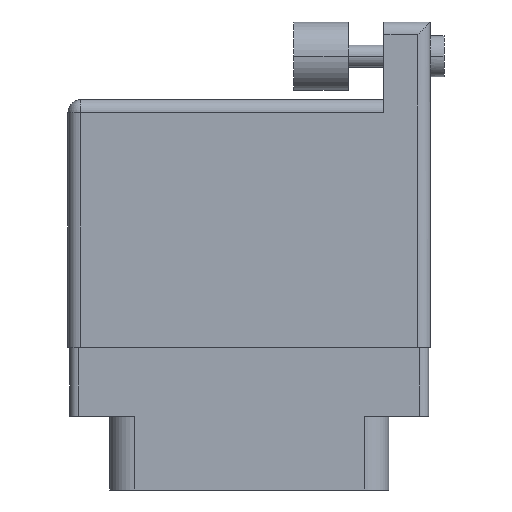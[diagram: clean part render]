
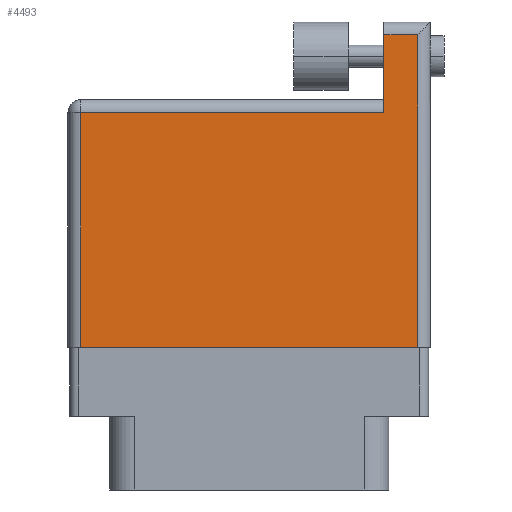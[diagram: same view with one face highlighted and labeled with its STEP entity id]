
A CAD part, front view. The second image highlights one B-rep face of the part: STEP entity #4493.
In plain terms, the highlighted face is planar.
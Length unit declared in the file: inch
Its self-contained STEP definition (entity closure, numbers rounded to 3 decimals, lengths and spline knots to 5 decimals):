
#418 = VECTOR ( 'NONE', #1665, 39.37008 ) ;
#433 = VERTEX_POINT ( 'NONE', #20289 ) ;
#471 = VECTOR ( 'NONE', #10760, 39.37008 ) ;
#1665 = DIRECTION ( 'NONE',  ( 0., 1., 0. ) ) ;
#1786 = CARTESIAN_POINT ( 'NONE',  ( 0.047, 0.859, 0. ) ) ;
#2271 = EDGE_CURVE ( 'NONE', #8817, #2777, #4031, .T. ) ;
#2643 = DIRECTION ( 'NONE',  ( 0., 0., -1. ) ) ;
#2777 = VERTEX_POINT ( 'NONE', #15949 ) ;
#2912 = VECTOR ( 'NONE', #10332, 39.37008 ) ;
#3326 = CARTESIAN_POINT ( 'NONE',  ( 1.278, 1.143, 0. ) ) ;
#3632 = ORIENTED_EDGE ( 'NONE', *, *, #8493, .T. ) ;
#4031 = LINE ( 'NONE', #20857, #2912 ) ;
#4182 = ORIENTED_EDGE ( 'NONE', *, *, #2271, .T. ) ;
#4493 = ADVANCED_FACE ( 'NONE', ( #7627 ), #17918, .F. ) ;
#5106 = LINE ( 'NONE', #11848, #418 ) ;
#5687 = ORIENTED_EDGE ( 'NONE', *, *, #17896, .T. ) ;
#5809 = LINE ( 'NONE', #12546, #18740 ) ;
#6690 = CARTESIAN_POINT ( 'NONE',  ( 1.155, 1.19, 0. ) ) ;
#7219 = CARTESIAN_POINT ( 'NONE',  ( 0.047, 0., 0. ) ) ;
#7345 = LINE ( 'NONE', #20630, #471 ) ;
#7584 = EDGE_LOOP ( 'NONE', ( #4182, #20610, #12353, #5687, #3632, #17560 ) ) ;
#7627 = FACE_OUTER_BOUND ( 'NONE', #7584, .T. ) ;
#8493 = EDGE_CURVE ( 'NONE', #10558, #19634, #5809, .T. ) ;
#8817 = VERTEX_POINT ( 'NONE', #7219 ) ;
#9152 = AXIS2_PLACEMENT_3D ( 'NONE', #15817, #2643, #10718 ) ;
#9871 = VERTEX_POINT ( 'NONE', #3326 ) ;
#10332 = DIRECTION ( 'NONE',  ( 1., 0., 0. ) ) ;
#10333 = VECTOR ( 'NONE', #11768, 39.37008 ) ;
#10558 = VERTEX_POINT ( 'NONE', #16752 ) ;
#10718 = DIRECTION ( 'NONE',  ( -1., 0., 0. ) ) ;
#10760 = DIRECTION ( 'NONE',  ( -1., 0., 0. ) ) ;
#11133 = EDGE_CURVE ( 'NONE', #2777, #9871, #5106, .T. ) ;
#11768 = DIRECTION ( 'NONE',  ( 0., -1., 0. ) ) ;
#11848 = CARTESIAN_POINT ( 'NONE',  ( 1.278, 1.19, 0. ) ) ;
#11880 = LINE ( 'NONE', #6690, #10333 ) ;
#12045 = CARTESIAN_POINT ( 'NONE',  ( 0.047, 0., 0. ) ) ;
#12353 = ORIENTED_EDGE ( 'NONE', *, *, #18096, .T. ) ;
#12546 = CARTESIAN_POINT ( 'NONE',  ( 0., 0.859, 0. ) ) ;
#15373 = LINE ( 'NONE', #12045, #18895 ) ;
#15579 = EDGE_CURVE ( 'NONE', #19634, #8817, #15373, .T. ) ;
#15817 = CARTESIAN_POINT ( 'NONE',  ( 0., 0.906, 0. ) ) ;
#15949 = CARTESIAN_POINT ( 'NONE',  ( 1.278, 0., 0. ) ) ;
#16752 = CARTESIAN_POINT ( 'NONE',  ( 1.155, 0.859, 0. ) ) ;
#17560 = ORIENTED_EDGE ( 'NONE', *, *, #15579, .T. ) ;
#17896 = EDGE_CURVE ( 'NONE', #433, #10558, #11880, .T. ) ;
#17918 = PLANE ( 'NONE',  #9152 ) ;
#18096 = EDGE_CURVE ( 'NONE', #9871, #433, #7345, .T. ) ;
#18740 = VECTOR ( 'NONE', #21185, 39.37008 ) ;
#18895 = VECTOR ( 'NONE', #21687, 39.37008 ) ;
#19634 = VERTEX_POINT ( 'NONE', #1786 ) ;
#20289 = CARTESIAN_POINT ( 'NONE',  ( 1.155, 1.143, 0. ) ) ;
#20610 = ORIENTED_EDGE ( 'NONE', *, *, #11133, .T. ) ;
#20630 = CARTESIAN_POINT ( 'NONE',  ( 1.155, 1.143, 0. ) ) ;
#20857 = CARTESIAN_POINT ( 'NONE',  ( 0., 0., 0. ) ) ;
#21185 = DIRECTION ( 'NONE',  ( -1., 0., 0. ) ) ;
#21687 = DIRECTION ( 'NONE',  ( 0., -1., 0. ) ) ;
